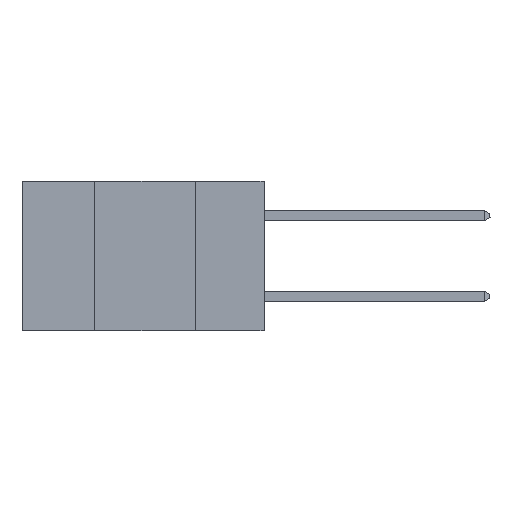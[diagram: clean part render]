
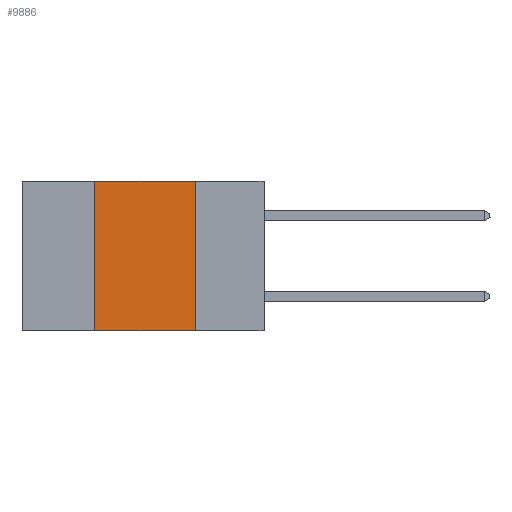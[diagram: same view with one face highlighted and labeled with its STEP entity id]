
A CAD part, left-side view. The second image highlights one B-rep face of the part: STEP entity #9886.
In plain terms, the highlighted planar face has unit normal (-1, 0, 0).
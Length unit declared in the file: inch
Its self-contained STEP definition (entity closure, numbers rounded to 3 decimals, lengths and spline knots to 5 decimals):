
#1437 = AXIS2_PLACEMENT_3D ( 'NONE', #9900, #17925, #7144 ) ;
#2306 = PLANE ( 'NONE',  #1437 ) ;
#2404 = DIRECTION ( 'NONE',  ( 0., 0., 1. ) ) ;
#2784 = CARTESIAN_POINT ( 'NONE',  ( 0., 0.42, -0.37 ) ) ;
#3283 = LINE ( 'NONE', #31082, #15602 ) ;
#5380 = DIRECTION ( 'NONE',  ( 0., -1., 0. ) ) ;
#6721 = CARTESIAN_POINT ( 'NONE',  ( 0., 0.42, 0. ) ) ;
#7144 = DIRECTION ( 'NONE',  ( 0., 0., -1. ) ) ;
#8279 = FACE_OUTER_BOUND ( 'NONE', #27723, .T. ) ;
#9804 = EDGE_CURVE ( 'NONE', #21637, #28404, #25087, .T. ) ;
#9886 = ADVANCED_FACE ( 'NONE', ( #8279 ), #2306, .F. ) ;
#9900 = CARTESIAN_POINT ( 'NONE',  ( 0., 0.6, 0. ) ) ;
#10665 = ORIENTED_EDGE ( 'NONE', *, *, #29393, .F. ) ;
#11572 = CARTESIAN_POINT ( 'NONE',  ( 0., 0.17, 0. ) ) ;
#13333 = LINE ( 'NONE', #11572, #30139 ) ;
#13973 = EDGE_CURVE ( 'NONE', #28404, #22388, #13333, .T. ) ;
#15602 = VECTOR ( 'NONE', #5380, 39.37008 ) ;
#17925 = DIRECTION ( 'NONE',  ( 1., 0., 0. ) ) ;
#18066 = LINE ( 'NONE', #18136, #28305 ) ;
#18136 = CARTESIAN_POINT ( 'NONE',  ( 0., 0.42, 0. ) ) ;
#20368 = CARTESIAN_POINT ( 'NONE',  ( 0., 0.17, -0.37 ) ) ;
#21637 = VERTEX_POINT ( 'NONE', #6721 ) ;
#22028 = ORIENTED_EDGE ( 'NONE', *, *, #29402, .T. ) ;
#22388 = VERTEX_POINT ( 'NONE', #20368 ) ;
#25087 = LINE ( 'NONE', #33803, #29184 ) ;
#25250 = DIRECTION ( 'NONE',  ( 0., 0., -1. ) ) ;
#26189 = VERTEX_POINT ( 'NONE', #2784 ) ;
#26348 = ORIENTED_EDGE ( 'NONE', *, *, #9804, .F. ) ;
#27723 = EDGE_LOOP ( 'NONE', ( #30302, #26348, #10665, #22028 ) ) ;
#28305 = VECTOR ( 'NONE', #2404, 39.37008 ) ;
#28404 = VERTEX_POINT ( 'NONE', #32373 ) ;
#29184 = VECTOR ( 'NONE', #33474, 39.37008 ) ;
#29393 = EDGE_CURVE ( 'NONE', #26189, #21637, #18066, .T. ) ;
#29402 = EDGE_CURVE ( 'NONE', #26189, #22388, #3283, .T. ) ;
#30139 = VECTOR ( 'NONE', #25250, 39.37008 ) ;
#30302 = ORIENTED_EDGE ( 'NONE', *, *, #13973, .F. ) ;
#31082 = CARTESIAN_POINT ( 'NONE',  ( 0., 0.6, -0.37 ) ) ;
#32373 = CARTESIAN_POINT ( 'NONE',  ( 0., 0.17, 0. ) ) ;
#33474 = DIRECTION ( 'NONE',  ( 0., -1., 0. ) ) ;
#33803 = CARTESIAN_POINT ( 'NONE',  ( 0., 0.6, 0. ) ) ;
